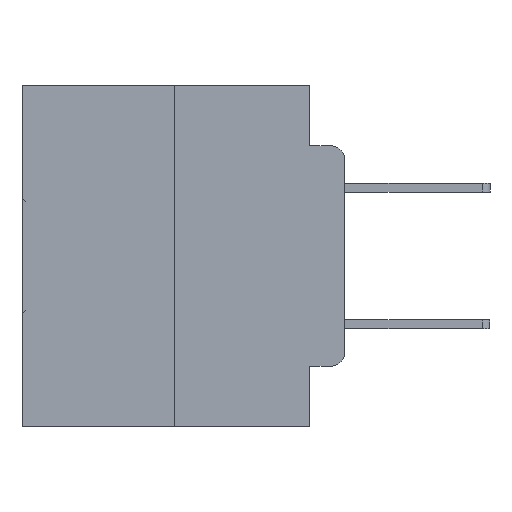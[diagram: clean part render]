
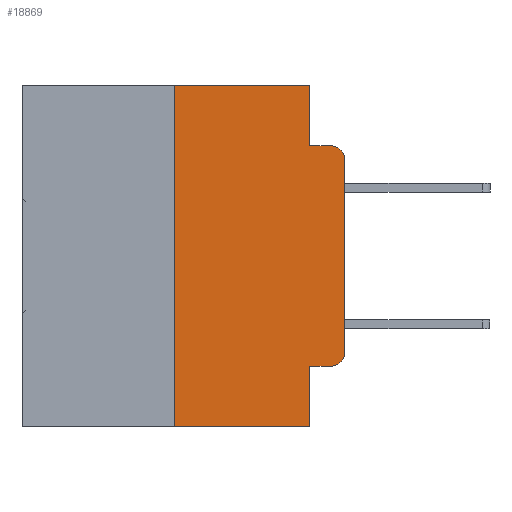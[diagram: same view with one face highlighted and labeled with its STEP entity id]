
A CAD part, left-side view. The second image highlights one B-rep face of the part: STEP entity #18869.
In plain terms, the highlighted planar face has unit normal (-1, 0, 0).
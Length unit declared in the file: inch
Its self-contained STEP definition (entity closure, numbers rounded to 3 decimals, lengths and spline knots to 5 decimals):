
#396 = LINE ( 'NONE', #16241, #26154 ) ;
#690 = AXIS2_PLACEMENT_3D ( 'NONE', #24603, #9378, #27096 ) ;
#998 = DIRECTION ( 'NONE',  ( -1., 0., 0. ) ) ;
#1307 = VECTOR ( 'NONE', #12861, 39.37008 ) ;
#1316 = VECTOR ( 'NONE', #5206, 39.37008 ) ;
#2715 = VERTEX_POINT ( 'NONE', #8673 ) ;
#3084 = ORIENTED_EDGE ( 'NONE', *, *, #12190, .F. ) ;
#3140 = VERTEX_POINT ( 'NONE', #7621 ) ;
#3400 = CARTESIAN_POINT ( 'NONE',  ( 0., 0., 0. ) ) ;
#3474 = EDGE_CURVE ( 'NONE', #3140, #24272, #25114, .T. ) ;
#3494 = LINE ( 'NONE', #11205, #16400 ) ;
#4174 = CARTESIAN_POINT ( 'NONE',  ( 0., 0.02, -0.1085 ) ) ;
#5194 = EDGE_CURVE ( 'NONE', #17228, #3140, #396, .T. ) ;
#5206 = DIRECTION ( 'NONE',  ( 0., -1., 0. ) ) ;
#5998 = CARTESIAN_POINT ( 'NONE',  ( 0., 0.051, -0.5 ) ) ;
#6315 = FACE_OUTER_BOUND ( 'NONE', #21061, .T. ) ;
#6480 = ORIENTED_EDGE ( 'NONE', *, *, #22410, .T. ) ;
#6745 = PLANE ( 'NONE',  #690 ) ;
#6812 = DIRECTION ( 'NONE',  ( 0., 0., -1. ) ) ;
#6935 = ORIENTED_EDGE ( 'NONE', *, *, #20737, .T. ) ;
#7440 = ORIENTED_EDGE ( 'NONE', *, *, #13905, .F. ) ;
#7621 = CARTESIAN_POINT ( 'NONE',  ( 0., 0.02, -0.4115 ) ) ;
#8604 = DIRECTION ( 'NONE',  ( 0., -1., 0. ) ) ;
#8673 = CARTESIAN_POINT ( 'NONE',  ( 0., 0.051, 0. ) ) ;
#8732 = EDGE_CURVE ( 'NONE', #17228, #26169, #8991, .T. ) ;
#8991 = LINE ( 'NONE', #17336, #14981 ) ;
#9113 = CARTESIAN_POINT ( 'NONE',  ( 0., 0.25, 0. ) ) ;
#9182 = AXIS2_PLACEMENT_3D ( 'NONE', #4174, #22139, #6812 ) ;
#9268 = VERTEX_POINT ( 'NONE', #11481 ) ;
#9378 = DIRECTION ( 'NONE',  ( 1., 0., 0. ) ) ;
#10483 = EDGE_CURVE ( 'NONE', #9268, #13176, #30645, .T. ) ;
#10950 = VERTEX_POINT ( 'NONE', #18655 ) ;
#11089 = VECTOR ( 'NONE', #17349, 39.37008 ) ;
#11126 = DIRECTION ( 'NONE',  ( 0., -1., 0. ) ) ;
#11205 = CARTESIAN_POINT ( 'NONE',  ( 0., 0.473, -0.5 ) ) ;
#11227 = ORIENTED_EDGE ( 'NONE', *, *, #10483, .F. ) ;
#11481 = CARTESIAN_POINT ( 'NONE',  ( 0., 0.25, -0.5 ) ) ;
#12190 = EDGE_CURVE ( 'NONE', #2715, #24156, #23478, .T. ) ;
#12861 = DIRECTION ( 'NONE',  ( 0., 0., -1. ) ) ;
#12877 = EDGE_CURVE ( 'NONE', #13176, #2715, #15153, .T. ) ;
#13044 = CARTESIAN_POINT ( 'NONE',  ( 0., 0.051, -0.0885 ) ) ;
#13176 = VERTEX_POINT ( 'NONE', #9113 ) ;
#13349 = ORIENTED_EDGE ( 'NONE', *, *, #5194, .T. ) ;
#13905 = EDGE_CURVE ( 'NONE', #24156, #27769, #24613, .T. ) ;
#14783 = CARTESIAN_POINT ( 'NONE',  ( 0., 0.051, -0.0885 ) ) ;
#14981 = VECTOR ( 'NONE', #27336, 39.37008 ) ;
#15153 = LINE ( 'NONE', #20745, #1316 ) ;
#16241 = CARTESIAN_POINT ( 'NONE',  ( 0., 0.051, -0.4115 ) ) ;
#16400 = VECTOR ( 'NONE', #8604, 39.37008 ) ;
#16566 = CARTESIAN_POINT ( 'NONE',  ( 0., 0.02, -0.3915 ) ) ;
#16888 = DIRECTION ( 'NONE',  ( 0., 0., 1. ) ) ;
#17228 = VERTEX_POINT ( 'NONE', #32798 ) ;
#17336 = CARTESIAN_POINT ( 'NONE',  ( 0., 0.051, 0. ) ) ;
#17349 = DIRECTION ( 'NONE',  ( 0., -1., 0. ) ) ;
#17883 = CARTESIAN_POINT ( 'NONE',  ( 0., 0.051, 0. ) ) ;
#18406 = ORIENTED_EDGE ( 'NONE', *, *, #12877, .F. ) ;
#18655 = CARTESIAN_POINT ( 'NONE',  ( 0., 0., -0.1085 ) ) ;
#18869 = ADVANCED_FACE ( 'NONE', ( #6315 ), #6745, .F. ) ;
#19157 = DIRECTION ( 'NONE',  ( 0., 0., -1. ) ) ;
#19534 = VECTOR ( 'NONE', #21385, 39.37008 ) ;
#20737 = EDGE_CURVE ( 'NONE', #10950, #27769, #28595, .T. ) ;
#20745 = CARTESIAN_POINT ( 'NONE',  ( 0., 0.473, 0. ) ) ;
#20954 = CARTESIAN_POINT ( 'NONE',  ( 0., 0.02, -0.0885 ) ) ;
#21061 = EDGE_LOOP ( 'NONE', ( #6480, #6935, #7440, #3084, #18406, #11227, #29073, #29107, #13349, #27200 ) ) ;
#21385 = DIRECTION ( 'NONE',  ( 0., 0., 1. ) ) ;
#21507 = CARTESIAN_POINT ( 'NONE',  ( 0., 0., -0.3915 ) ) ;
#22139 = DIRECTION ( 'NONE',  ( -1., 0., 0. ) ) ;
#22410 = EDGE_CURVE ( 'NONE', #24272, #10950, #32069, .T. ) ;
#23478 = LINE ( 'NONE', #17883, #1307 ) ;
#24156 = VERTEX_POINT ( 'NONE', #13044 ) ;
#24272 = VERTEX_POINT ( 'NONE', #21507 ) ;
#24603 = CARTESIAN_POINT ( 'NONE',  ( 0., 0.473, 0. ) ) ;
#24613 = LINE ( 'NONE', #14783, #11089 ) ;
#25114 = CIRCLE ( 'NONE', #31761, 0.02 ) ;
#26154 = VECTOR ( 'NONE', #11126, 39.37008 ) ;
#26169 = VERTEX_POINT ( 'NONE', #5998 ) ;
#26626 = EDGE_CURVE ( 'NONE', #9268, #26169, #3494, .T. ) ;
#26898 = CARTESIAN_POINT ( 'NONE',  ( 0., 0.25, 0. ) ) ;
#27096 = DIRECTION ( 'NONE',  ( 0., 0., -1. ) ) ;
#27200 = ORIENTED_EDGE ( 'NONE', *, *, #3474, .T. ) ;
#27336 = DIRECTION ( 'NONE',  ( 0., 0., -1. ) ) ;
#27769 = VERTEX_POINT ( 'NONE', #20954 ) ;
#28595 = CIRCLE ( 'NONE', #9182, 0.02 ) ;
#29073 = ORIENTED_EDGE ( 'NONE', *, *, #26626, .T. ) ;
#29107 = ORIENTED_EDGE ( 'NONE', *, *, #8732, .F. ) ;
#29861 = VECTOR ( 'NONE', #16888, 39.37008 ) ;
#30645 = LINE ( 'NONE', #26898, #29861 ) ;
#31761 = AXIS2_PLACEMENT_3D ( 'NONE', #16566, #998, #19157 ) ;
#32069 = LINE ( 'NONE', #3400, #19534 ) ;
#32798 = CARTESIAN_POINT ( 'NONE',  ( 0., 0.051, -0.4115 ) ) ;
